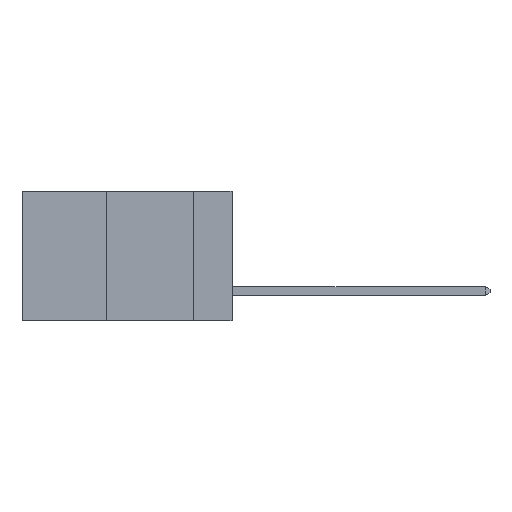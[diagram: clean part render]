
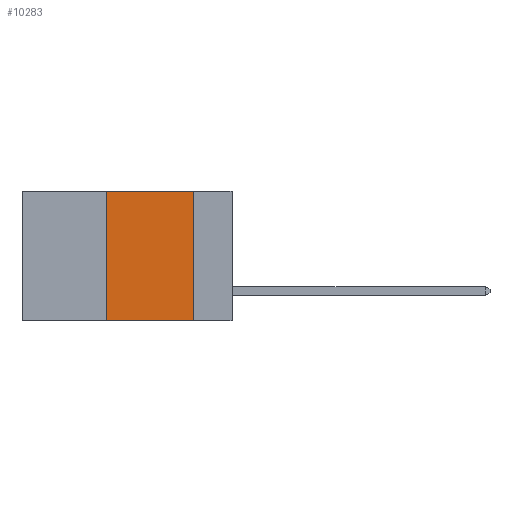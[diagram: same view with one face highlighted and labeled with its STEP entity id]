
A CAD part, left-side view. The second image highlights one B-rep face of the part: STEP entity #10283.
In plain terms, the highlighted planar face has unit normal (-1, 0, 0).
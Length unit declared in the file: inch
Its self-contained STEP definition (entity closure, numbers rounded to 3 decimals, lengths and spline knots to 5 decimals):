
#125 = VERTEX_POINT ( 'NONE', #10840 ) ;
#1072 = DIRECTION ( 'NONE',  ( 1., 0., 0. ) ) ;
#1126 = DIRECTION ( 'NONE',  ( 0., -1., 0. ) ) ;
#1519 = LINE ( 'NONE', #14045, #4821 ) ;
#1558 = ORIENTED_EDGE ( 'NONE', *, *, #4644, .T. ) ;
#2633 = EDGE_LOOP ( 'NONE', ( #13670, #7458, #14405, #1558 ) ) ;
#3118 = DIRECTION ( 'NONE',  ( 0., 0., 1. ) ) ;
#3150 = AXIS2_PLACEMENT_3D ( 'NONE', #8602, #1072, #9860 ) ;
#3400 = VERTEX_POINT ( 'NONE', #16048 ) ;
#4644 = EDGE_CURVE ( 'NONE', #125, #3400, #1519, .T. ) ;
#4821 = VECTOR ( 'NONE', #1126, 39.37008 ) ;
#5214 = EDGE_CURVE ( 'NONE', #5886, #11402, #15637, .T. ) ;
#5886 = VERTEX_POINT ( 'NONE', #15657 ) ;
#6924 = DIRECTION ( 'NONE',  ( 0., -1., 0. ) ) ;
#7245 = CARTESIAN_POINT ( 'NONE',  ( 0., 0.6, 0. ) ) ;
#7458 = ORIENTED_EDGE ( 'NONE', *, *, #5214, .F. ) ;
#8066 = CARTESIAN_POINT ( 'NONE',  ( 0., 0.36, 0. ) ) ;
#8342 = FACE_OUTER_BOUND ( 'NONE', #2633, .T. ) ;
#8602 = CARTESIAN_POINT ( 'NONE',  ( 0., 0.6, 0. ) ) ;
#8791 = VECTOR ( 'NONE', #3118, 39.37008 ) ;
#9206 = LINE ( 'NONE', #9647, #14931 ) ;
#9647 = CARTESIAN_POINT ( 'NONE',  ( 0., 0.11, 0. ) ) ;
#9860 = DIRECTION ( 'NONE',  ( 0., 0., -1. ) ) ;
#10283 = ADVANCED_FACE ( 'NONE', ( #8342 ), #15899, .F. ) ;
#10840 = CARTESIAN_POINT ( 'NONE',  ( 0., 0.36, -0.37 ) ) ;
#11402 = VERTEX_POINT ( 'NONE', #14475 ) ;
#12478 = VECTOR ( 'NONE', #6924, 39.37008 ) ;
#13394 = DIRECTION ( 'NONE',  ( 0., 0., -1. ) ) ;
#13670 = ORIENTED_EDGE ( 'NONE', *, *, #14936, .F. ) ;
#14045 = CARTESIAN_POINT ( 'NONE',  ( 0., 0.6, -0.37 ) ) ;
#14405 = ORIENTED_EDGE ( 'NONE', *, *, #15731, .F. ) ;
#14475 = CARTESIAN_POINT ( 'NONE',  ( 0., 0.11, 0. ) ) ;
#14931 = VECTOR ( 'NONE', #13394, 39.37008 ) ;
#14936 = EDGE_CURVE ( 'NONE', #11402, #3400, #9206, .T. ) ;
#15283 = LINE ( 'NONE', #8066, #8791 ) ;
#15637 = LINE ( 'NONE', #7245, #12478 ) ;
#15657 = CARTESIAN_POINT ( 'NONE',  ( 0., 0.36, 0. ) ) ;
#15731 = EDGE_CURVE ( 'NONE', #125, #5886, #15283, .T. ) ;
#15899 = PLANE ( 'NONE',  #3150 ) ;
#16048 = CARTESIAN_POINT ( 'NONE',  ( 0., 0.11, -0.37 ) ) ;
